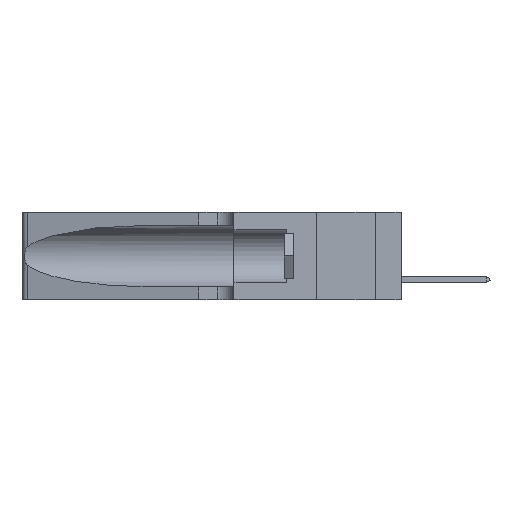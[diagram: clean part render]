
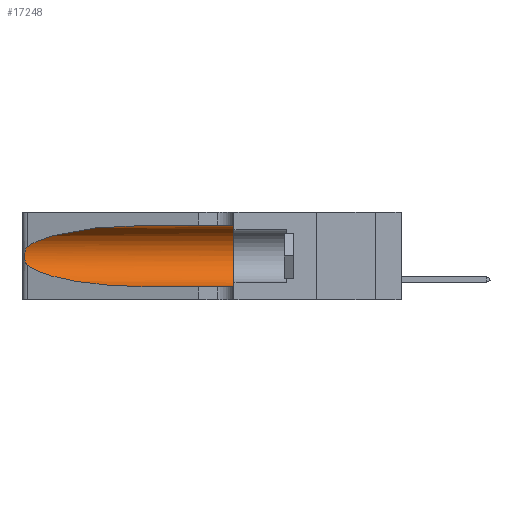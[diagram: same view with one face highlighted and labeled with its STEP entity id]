
A CAD part, left-side view. The second image highlights one B-rep face of the part: STEP entity #17248.
In plain terms, the highlighted cylindrical face has radius 3.308 mm (diameter 6.617 mm), a partial arc.
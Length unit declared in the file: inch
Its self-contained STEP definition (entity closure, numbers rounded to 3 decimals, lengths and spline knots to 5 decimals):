
#2050 = ORIENTED_EDGE ( 'NONE', *, *, #38617, .T. ) ;
#2378 = CARTESIAN_POINT ( 'NONE',  ( 0.2373, 1.15595, 0.08982 ) ) ;
#2416 = ORIENTED_EDGE ( 'NONE', *, *, #6404, .T. ) ;
#2778 = CARTESIAN_POINT ( 'NONE',  ( 0.25854, 1.2359, 0.20912 ) ) ;
#3415 = CARTESIAN_POINT ( 'NONE',  ( 0.1305, 0.35, 0.31525 ) ) ;
#4739 = ORIENTED_EDGE ( 'NONE', *, *, #8968, .F. ) ;
#6283 = CARTESIAN_POINT ( 'NONE',  ( 0.25856, 1.23593, 0.16098 ) ) ;
#6404 = EDGE_CURVE ( 'NONE', #12585, #37941, #31253, .T. ) ;
#6455 = CARTESIAN_POINT ( 'NONE',  ( 0.25639, 1.23186, 0.15144 ) ) ;
#6634 = CARTESIAN_POINT ( 'NONE',  ( 0.26018, 1.23835, 0.19895 ) ) ;
#6641 = CARTESIAN_POINT ( 'NONE',  ( 0.1305, 0.35, 0.185 ) ) ;
#7458 = CARTESIAN_POINT ( 'NONE',  ( 0.25487, 1.22718, 0.22369 ) ) ;
#7966 = AXIS2_PLACEMENT_3D ( 'NONE', #9638, #48345, #25343 ) ;
#8968 = EDGE_CURVE ( 'NONE', #12585, #17999, #42654, .T. ) ;
#9638 = CARTESIAN_POINT ( 'NONE',  ( 0.1305, 1.61858, 0.185 ) ) ;
#9883 = EDGE_CURVE ( 'NONE', #17999, #24573, #46763, .T. ) ;
#10132 = CARTESIAN_POINT ( 'NONE',  ( 0.1305, 1.61858, 0.05475 ) ) ;
#11799 = EDGE_CURVE ( 'NONE', #23360, #32305, #26888, .T. ) ;
#12585 = VERTEX_POINT ( 'NONE', #25206 ) ;
#13103 = EDGE_LOOP ( 'NONE', ( #2416, #25023, #42707, #2050, #25687, #4739 ) ) ;
#14560 = CARTESIAN_POINT ( 'NONE',  ( 0.26075, 1.23896, 0.19203 ) ) ;
#15506 = CYLINDRICAL_SURFACE ( 'NONE', #7966, 0.13025 ) ;
#16913 = CARTESIAN_POINT ( 'NONE',  ( 0.1305, 0.72297, 0.31525 ) ) ;
#17248 = ADVANCED_FACE ( 'NONE', ( #44502 ), #15506, .F. ) ;
#17999 = VERTEX_POINT ( 'NONE', #3415 ) ;
#19034 = VECTOR ( 'NONE', #29511, 39.37008 ) ;
#20840 = CARTESIAN_POINT ( 'NONE',  ( 0.1305, 0.72297, 0.05475 ) ) ;
#22103 = CARTESIAN_POINT ( 'NONE',  ( 0.25555, 1.22994, 0.2215 ) ) ;
#22215 = EDGE_CURVE ( 'NONE', #37941, #23360, #22883, .T. ) ;
#22630 = VECTOR ( 'NONE', #29420, 39.37008 ) ;
#22883 = B_SPLINE_CURVE_WITH_KNOTS ( 'NONE', 3,
 ( #49037, #22103, #49201, #25860, #2778, #6634, #14560, #29777, #41604, #6283, #29430, #6455, #26027, #29955 ),
 .UNSPECIFIED., .F., .F.,
 ( 4, 2, 2, 2, 2, 2, 4 ),
 ( 0., 0.00027, 0.00053, 0.00107, 0.0016, 0.00187, 0.00214 ),
 .UNSPECIFIED. ) ;
#23360 = VERTEX_POINT ( 'NONE', #35505 ) ;
#24033 = DIRECTION ( 'NONE',  ( 0., 1., 0. ) ) ;
#24573 = VERTEX_POINT ( 'NONE', #30760 ) ;
#25023 = ORIENTED_EDGE ( 'NONE', *, *, #22215, .T. ) ;
#25206 = CARTESIAN_POINT ( 'NONE',  ( 0.1305, 0.72297, 0.31525 ) ) ;
#25343 = DIRECTION ( 'NONE',  ( 0., 0., -1. ) ) ;
#25687 = ORIENTED_EDGE ( 'NONE', *, *, #9883, .F. ) ;
#25790 = DIRECTION ( 'NONE',  ( 0., 0., 1. ) ) ;
#25860 = CARTESIAN_POINT ( 'NONE',  ( 0.25787, 1.23484, 0.2124 ) ) ;
#25909 = CARTESIAN_POINT ( 'NONE',  ( 0.2373, 1.15595, 0.28018 ) ) ;
#26027 = CARTESIAN_POINT ( 'NONE',  ( 0.25555, 1.22993, 0.14849 ) ) ;
#26888 =( BOUNDED_CURVE ( )  B_SPLINE_CURVE ( 3, ( #33279, #2378, #44176, #40838 ),
 .UNSPECIFIED., .F., .T. ) 
 B_SPLINE_CURVE_WITH_KNOTS ( ( 4, 4 ),
 ( 3.44316, 4.71239 ),
 .UNSPECIFIED. ) 
 CURVE ( )  GEOMETRIC_REPRESENTATION_ITEM ( )  RATIONAL_B_SPLINE_CURVE ( ( 1., 0.87, 0.87, 1. ) ) 
 REPRESENTATION_ITEM ( '' )  );
#29420 = DIRECTION ( 'NONE',  ( 0., -1., 0. ) ) ;
#29430 = CARTESIAN_POINT ( 'NONE',  ( 0.25789, 1.23486, 0.15765 ) ) ;
#29511 = DIRECTION ( 'NONE',  ( 0., -1., 0. ) ) ;
#29777 = CARTESIAN_POINT ( 'NONE',  ( 0.26075, 1.23896, 0.178 ) ) ;
#29955 = CARTESIAN_POINT ( 'NONE',  ( 0.25487, 1.22718, 0.14631 ) ) ;
#30760 = CARTESIAN_POINT ( 'NONE',  ( 0.1305, 0.35, 0.05475 ) ) ;
#31253 =( BOUNDED_CURVE ( )  B_SPLINE_CURVE ( 3, ( #16913, #49641, #25909, #7458 ),
 .UNSPECIFIED., .F., .T. ) 
 B_SPLINE_CURVE_WITH_KNOTS ( ( 4, 4 ),
 ( 1.5708, 2.84003 ),
 .UNSPECIFIED. ) 
 CURVE ( )  GEOMETRIC_REPRESENTATION_ITEM ( )  RATIONAL_B_SPLINE_CURVE ( ( 1., 0.87, 0.87, 1. ) ) 
 REPRESENTATION_ITEM ( '' )  );
#32305 = VERTEX_POINT ( 'NONE', #20840 ) ;
#32861 = CARTESIAN_POINT ( 'NONE',  ( 0.1305, 1.61858, 0.31525 ) ) ;
#33279 = CARTESIAN_POINT ( 'NONE',  ( 0.25487, 1.22718, 0.14631 ) ) ;
#35505 = CARTESIAN_POINT ( 'NONE',  ( 0.25487, 1.22718, 0.14631 ) ) ;
#35879 = LINE ( 'NONE', #10132, #22630 ) ;
#36881 = CARTESIAN_POINT ( 'NONE',  ( 0.25487, 1.22718, 0.22369 ) ) ;
#37941 = VERTEX_POINT ( 'NONE', #36881 ) ;
#38617 = EDGE_CURVE ( 'NONE', #32305, #24573, #35879, .T. ) ;
#40288 = AXIS2_PLACEMENT_3D ( 'NONE', #6641, #24033, #25790 ) ;
#40838 = CARTESIAN_POINT ( 'NONE',  ( 0.1305, 0.72297, 0.05475 ) ) ;
#41604 = CARTESIAN_POINT ( 'NONE',  ( 0.26017, 1.23833, 0.17102 ) ) ;
#42654 = LINE ( 'NONE', #32861, #19034 ) ;
#42707 = ORIENTED_EDGE ( 'NONE', *, *, #11799, .T. ) ;
#44176 = CARTESIAN_POINT ( 'NONE',  ( 0.18966, 0.96281, 0.05475 ) ) ;
#44502 = FACE_OUTER_BOUND ( 'NONE', #13103, .T. ) ;
#46763 = CIRCLE ( 'NONE', #40288, 0.13025 ) ;
#48345 = DIRECTION ( 'NONE',  ( 0., -1., 0. ) ) ;
#49037 = CARTESIAN_POINT ( 'NONE',  ( 0.25487, 1.22718, 0.22369 ) ) ;
#49201 = CARTESIAN_POINT ( 'NONE',  ( 0.25639, 1.23184, 0.21858 ) ) ;
#49641 = CARTESIAN_POINT ( 'NONE',  ( 0.18966, 0.96281, 0.31525 ) ) ;
